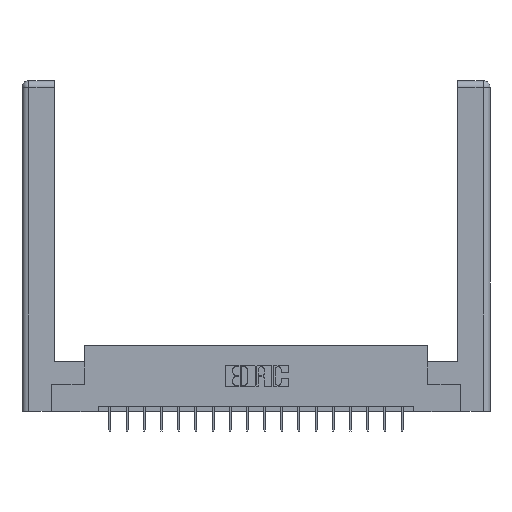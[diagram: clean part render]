
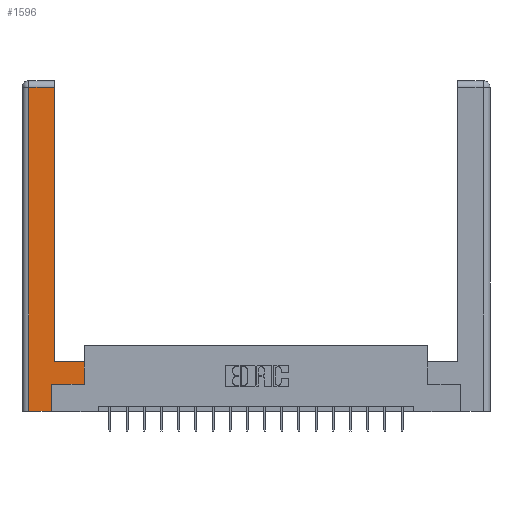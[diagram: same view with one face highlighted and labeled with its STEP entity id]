
A CAD part, top view. The second image highlights one B-rep face of the part: STEP entity #1596.
In plain terms, the highlighted planar face has unit normal (0, 0, 1).
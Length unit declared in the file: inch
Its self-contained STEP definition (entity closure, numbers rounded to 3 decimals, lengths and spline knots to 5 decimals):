
#227 = ORIENTED_EDGE ( 'NONE', *, *, #15797, .T. ) ;
#261 = CARTESIAN_POINT ( 'NONE',  ( 0.0615, 2.94, 0. ) ) ;
#657 = EDGE_CURVE ( 'NONE', #15077, #13753, #3277, .T. ) ;
#703 = CARTESIAN_POINT ( 'NONE',  ( 0.0615, 2.94, 0. ) ) ;
#1596 = ADVANCED_FACE ( 'NONE', ( #2771 ), #2721, .F. ) ;
#1608 = DIRECTION ( 'NONE',  ( 0., 1., 0. ) ) ;
#1851 = VERTEX_POINT ( 'NONE', #6485 ) ;
#2002 = LINE ( 'NONE', #6641, #13716 ) ;
#2110 = ORIENTED_EDGE ( 'NONE', *, *, #7457, .T. ) ;
#2372 = CARTESIAN_POINT ( 'NONE',  ( 0.565, 0.245, 0. ) ) ;
#2419 = ORIENTED_EDGE ( 'NONE', *, *, #2479, .T. ) ;
#2426 = VERTEX_POINT ( 'NONE', #12561 ) ;
#2479 = EDGE_CURVE ( 'NONE', #12599, #1851, #12775, .T. ) ;
#2721 = PLANE ( 'NONE',  #16052 ) ;
#2771 = FACE_OUTER_BOUND ( 'NONE', #6040, .T. ) ;
#2860 = EDGE_CURVE ( 'NONE', #4132, #2426, #15787, .T. ) ;
#3277 = LINE ( 'NONE', #19278, #17872 ) ;
#3318 = ORIENTED_EDGE ( 'NONE', *, *, #5812, .T. ) ;
#3473 = CARTESIAN_POINT ( 'NONE',  ( 0.265, 0., 0. ) ) ;
#4132 = VERTEX_POINT ( 'NONE', #2372 ) ;
#4233 = CARTESIAN_POINT ( 'NONE',  ( 0., 0., 0. ) ) ;
#4438 = LINE ( 'NONE', #8033, #8969 ) ;
#4648 = ORIENTED_EDGE ( 'NONE', *, *, #657, .T. ) ;
#5003 = VECTOR ( 'NONE', #18084, 39.37008 ) ;
#5591 = ORIENTED_EDGE ( 'NONE', *, *, #11735, .T. ) ;
#5812 = EDGE_CURVE ( 'NONE', #1851, #15077, #16828, .T. ) ;
#6040 = EDGE_LOOP ( 'NONE', ( #2110, #5591, #2419, #3318, #4648, #16750, #16024, #227 ) ) ;
#6485 = CARTESIAN_POINT ( 'NONE',  ( 0.0615, 0., 0. ) ) ;
#6641 = CARTESIAN_POINT ( 'NONE',  ( 0.295, 0.45, 0. ) ) ;
#7457 = EDGE_CURVE ( 'NONE', #13718, #8315, #10334, .T. ) ;
#7534 = VECTOR ( 'NONE', #12507, 39.37008 ) ;
#8020 = LINE ( 'NONE', #261, #7534 ) ;
#8033 = CARTESIAN_POINT ( 'NONE',  ( 0.565, 0.245, 0. ) ) ;
#8315 = VERTEX_POINT ( 'NONE', #8560 ) ;
#8560 = CARTESIAN_POINT ( 'NONE',  ( 0.295, 2.94, 0. ) ) ;
#8668 = CARTESIAN_POINT ( 'NONE',  ( 0.265, 0., 0. ) ) ;
#8969 = VECTOR ( 'NONE', #18457, 39.37008 ) ;
#9176 = CARTESIAN_POINT ( 'NONE',  ( 0.265, 0.245, 0. ) ) ;
#9203 = CARTESIAN_POINT ( 'NONE',  ( 0.295, 3., 0. ) ) ;
#10334 = LINE ( 'NONE', #9203, #16797 ) ;
#10364 = DIRECTION ( 'NONE',  ( -1., 0., 0. ) ) ;
#10623 = EDGE_CURVE ( 'NONE', #13753, #4132, #4438, .T. ) ;
#11037 = DIRECTION ( 'NONE',  ( 0., -1., 0. ) ) ;
#11674 = DIRECTION ( 'NONE',  ( 0., 1., 0. ) ) ;
#11735 = EDGE_CURVE ( 'NONE', #8315, #12599, #8020, .T. ) ;
#11797 = VECTOR ( 'NONE', #11037, 39.37008 ) ;
#11883 = CARTESIAN_POINT ( 'NONE',  ( 0.565, 0.45, 0. ) ) ;
#12310 = VECTOR ( 'NONE', #17189, 39.37008 ) ;
#12507 = DIRECTION ( 'NONE',  ( -1., 0., 0. ) ) ;
#12561 = CARTESIAN_POINT ( 'NONE',  ( 0.565, 0.45, 0. ) ) ;
#12599 = VERTEX_POINT ( 'NONE', #703 ) ;
#12775 = LINE ( 'NONE', #14223, #11797 ) ;
#13426 = CARTESIAN_POINT ( 'NONE',  ( 0.295, 0.45, 0. ) ) ;
#13716 = VECTOR ( 'NONE', #15800, 39.37008 ) ;
#13718 = VERTEX_POINT ( 'NONE', #13426 ) ;
#13753 = VERTEX_POINT ( 'NONE', #9176 ) ;
#14223 = CARTESIAN_POINT ( 'NONE',  ( 0.0615, 0., 0. ) ) ;
#15077 = VERTEX_POINT ( 'NONE', #8668 ) ;
#15787 = LINE ( 'NONE', #11883, #5003 ) ;
#15797 = EDGE_CURVE ( 'NONE', #2426, #13718, #2002, .T. ) ;
#15800 = DIRECTION ( 'NONE',  ( -1., 0., 0. ) ) ;
#16024 = ORIENTED_EDGE ( 'NONE', *, *, #2860, .T. ) ;
#16052 = AXIS2_PLACEMENT_3D ( 'NONE', #4233, #19519, #10364 ) ;
#16750 = ORIENTED_EDGE ( 'NONE', *, *, #10623, .T. ) ;
#16797 = VECTOR ( 'NONE', #1608, 39.37008 ) ;
#16828 = LINE ( 'NONE', #3473, #12310 ) ;
#17189 = DIRECTION ( 'NONE',  ( 1., 0., 0. ) ) ;
#17872 = VECTOR ( 'NONE', #11674, 39.37008 ) ;
#18084 = DIRECTION ( 'NONE',  ( 0., 1., 0. ) ) ;
#18457 = DIRECTION ( 'NONE',  ( 1., 0., 0. ) ) ;
#19278 = CARTESIAN_POINT ( 'NONE',  ( 0.265, 0.245, 0. ) ) ;
#19519 = DIRECTION ( 'NONE',  ( 0., 0., -1. ) ) ;
